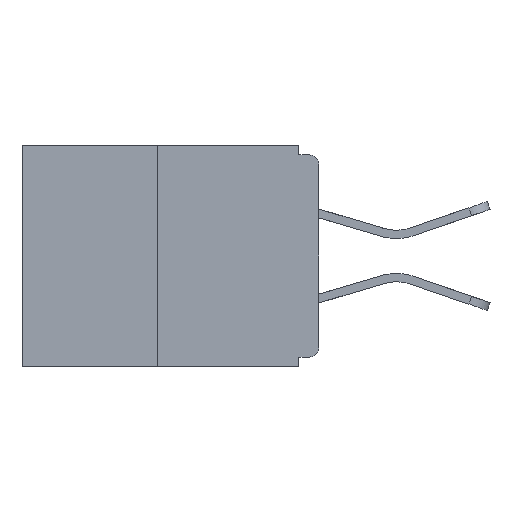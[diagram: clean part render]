
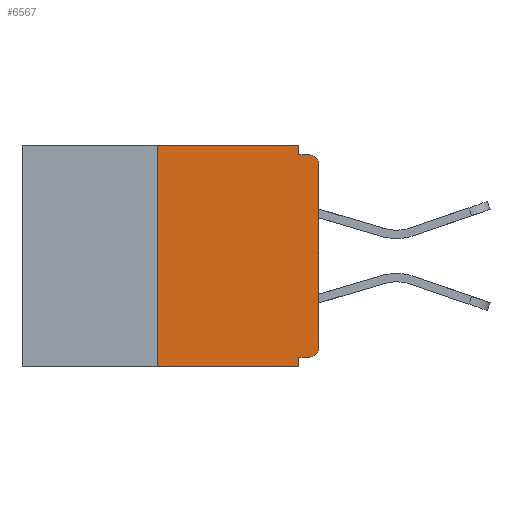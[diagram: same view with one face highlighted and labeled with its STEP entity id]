
A CAD part, left-side view. The second image highlights one B-rep face of the part: STEP entity #6567.
In plain terms, the highlighted planar face has unit normal (-1, 0, 0).
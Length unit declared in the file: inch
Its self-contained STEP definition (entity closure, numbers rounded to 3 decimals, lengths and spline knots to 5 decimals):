
#569 = LINE ( 'NONE', #5429, #4972 ) ;
#860 = LINE ( 'NONE', #4006, #21676 ) ;
#895 = AXIS2_PLACEMENT_3D ( 'NONE', #10374, #14402, #15822 ) ;
#920 = CARTESIAN_POINT ( 'NONE',  ( 0., 0.015, -0.328 ) ) ;
#1297 = ORIENTED_EDGE ( 'NONE', *, *, #5901, .F. ) ;
#1322 = DIRECTION ( 'NONE',  ( 0., 1., 0. ) ) ;
#1736 = DIRECTION ( 'NONE',  ( 0., -1., 0. ) ) ;
#2370 = CARTESIAN_POINT ( 'NONE',  ( 0., 0.031, -0.343 ) ) ;
#2407 = DIRECTION ( 'NONE',  ( 0., 0., 1. ) ) ;
#3159 = ORIENTED_EDGE ( 'NONE', *, *, #17744, .T. ) ;
#3407 = VERTEX_POINT ( 'NONE', #920 ) ;
#3622 = CARTESIAN_POINT ( 'NONE',  ( 0., 0.46, 0. ) ) ;
#4006 = CARTESIAN_POINT ( 'NONE',  ( 0., 0., -0.015 ) ) ;
#4726 = LINE ( 'NONE', #2370, #10388 ) ;
#4780 = CARTESIAN_POINT ( 'NONE',  ( 0., 0.031, -0.328 ) ) ;
#4972 = VECTOR ( 'NONE', #25666, 39.37008 ) ;
#5209 = VERTEX_POINT ( 'NONE', #5967 ) ;
#5330 = ORIENTED_EDGE ( 'NONE', *, *, #9795, .F. ) ;
#5429 = CARTESIAN_POINT ( 'NONE',  ( 0., 0., 0. ) ) ;
#5585 = LINE ( 'NONE', #11495, #7769 ) ;
#5897 = DIRECTION ( 'NONE',  ( 0., -1., 0. ) ) ;
#5901 = EDGE_CURVE ( 'NONE', #5209, #8011, #860, .T. ) ;
#5967 = CARTESIAN_POINT ( 'NONE',  ( 0., 0.031, -0.015 ) ) ;
#6097 = CARTESIAN_POINT ( 'NONE',  ( 0., 0.015, -0.015 ) ) ;
#6567 = ADVANCED_FACE ( 'NONE', ( #22589 ), #18854, .F. ) ;
#6778 = ORIENTED_EDGE ( 'NONE', *, *, #25465, .F. ) ;
#7506 = ORIENTED_EDGE ( 'NONE', *, *, #18424, .F. ) ;
#7606 = AXIS2_PLACEMENT_3D ( 'NONE', #22910, #8778, #23090 ) ;
#7614 = EDGE_CURVE ( 'NONE', #8412, #9125, #20313, .T. ) ;
#7769 = VECTOR ( 'NONE', #21606, 39.37008 ) ;
#8011 = VERTEX_POINT ( 'NONE', #6097 ) ;
#8253 = ORIENTED_EDGE ( 'NONE', *, *, #10452, .F. ) ;
#8412 = VERTEX_POINT ( 'NONE', #9722 ) ;
#8778 = DIRECTION ( 'NONE',  ( 1., 0., 0. ) ) ;
#8795 = CARTESIAN_POINT ( 'NONE',  ( 0., 0.25, 0. ) ) ;
#8951 = CARTESIAN_POINT ( 'NONE',  ( 0., 0.031, 0. ) ) ;
#9125 = VERTEX_POINT ( 'NONE', #23858 ) ;
#9319 = VECTOR ( 'NONE', #1322, 39.37008 ) ;
#9512 = VERTEX_POINT ( 'NONE', #4780 ) ;
#9722 = CARTESIAN_POINT ( 'NONE',  ( 0., 0.25, -0.343 ) ) ;
#9795 = EDGE_CURVE ( 'NONE', #9125, #11968, #23371, .T. ) ;
#10374 = CARTESIAN_POINT ( 'NONE',  ( 0., 0.015, -0.313 ) ) ;
#10388 = VECTOR ( 'NONE', #18570, 39.37008 ) ;
#10452 = EDGE_CURVE ( 'NONE', #9512, #11404, #4726, .T. ) ;
#10732 = CARTESIAN_POINT ( 'NONE',  ( 0., 0., -0.328 ) ) ;
#11404 = VERTEX_POINT ( 'NONE', #15299 ) ;
#11495 = CARTESIAN_POINT ( 'NONE',  ( 0., 0.031, 0. ) ) ;
#11968 = VERTEX_POINT ( 'NONE', #8951 ) ;
#12289 = ORIENTED_EDGE ( 'NONE', *, *, #17236, .T. ) ;
#13171 = CIRCLE ( 'NONE', #16526, 0.015 ) ;
#13923 = CARTESIAN_POINT ( 'NONE',  ( 0., 0., -0.03 ) ) ;
#14402 = DIRECTION ( 'NONE',  ( -1., 0., 0. ) ) ;
#14895 = EDGE_CURVE ( 'NONE', #14925, #8011, #13171, .T. ) ;
#14925 = VERTEX_POINT ( 'NONE', #13923 ) ;
#15299 = CARTESIAN_POINT ( 'NONE',  ( 0., 0.031, -0.343 ) ) ;
#15401 = DIRECTION ( 'NONE',  ( 0., -1., 0. ) ) ;
#15443 = VECTOR ( 'NONE', #5897, 39.37008 ) ;
#15592 = ORIENTED_EDGE ( 'NONE', *, *, #7614, .F. ) ;
#15805 = DIRECTION ( 'NONE',  ( -1., 0., 0. ) ) ;
#15822 = DIRECTION ( 'NONE',  ( 0., 0., -1. ) ) ;
#16526 = AXIS2_PLACEMENT_3D ( 'NONE', #18045, #15805, #19916 ) ;
#17236 = EDGE_CURVE ( 'NONE', #3407, #22325, #20793, .T. ) ;
#17744 = EDGE_CURVE ( 'NONE', #22325, #14925, #569, .T. ) ;
#18045 = CARTESIAN_POINT ( 'NONE',  ( 0., 0.015, -0.03 ) ) ;
#18424 = EDGE_CURVE ( 'NONE', #3407, #9512, #19757, .T. ) ;
#18570 = DIRECTION ( 'NONE',  ( 0., 0., -1. ) ) ;
#18854 = PLANE ( 'NONE',  #7606 ) ;
#19009 = VECTOR ( 'NONE', #2407, 39.37008 ) ;
#19250 = CARTESIAN_POINT ( 'NONE',  ( 0., 0., -0.313 ) ) ;
#19757 = LINE ( 'NONE', #10732, #9319 ) ;
#19842 = ORIENTED_EDGE ( 'NONE', *, *, #22861, .T. ) ;
#19894 = EDGE_LOOP ( 'NONE', ( #5330, #15592, #19842, #8253, #7506, #12289, #3159, #21653, #1297, #6778 ) ) ;
#19916 = DIRECTION ( 'NONE',  ( 0., 0., -1. ) ) ;
#20313 = LINE ( 'NONE', #8795, #19009 ) ;
#20793 = CIRCLE ( 'NONE', #895, 0.015 ) ;
#21606 = DIRECTION ( 'NONE',  ( 0., 0., -1. ) ) ;
#21653 = ORIENTED_EDGE ( 'NONE', *, *, #14895, .T. ) ;
#21676 = VECTOR ( 'NONE', #1736, 39.37008 ) ;
#22325 = VERTEX_POINT ( 'NONE', #19250 ) ;
#22589 = FACE_OUTER_BOUND ( 'NONE', #19894, .T. ) ;
#22861 = EDGE_CURVE ( 'NONE', #8412, #11404, #22991, .T. ) ;
#22910 = CARTESIAN_POINT ( 'NONE',  ( 0., 0.46, 0. ) ) ;
#22991 = LINE ( 'NONE', #25346, #25225 ) ;
#23090 = DIRECTION ( 'NONE',  ( 0., 0., -1. ) ) ;
#23371 = LINE ( 'NONE', #3622, #15443 ) ;
#23858 = CARTESIAN_POINT ( 'NONE',  ( 0., 0.25, 0. ) ) ;
#25225 = VECTOR ( 'NONE', #15401, 39.37008 ) ;
#25346 = CARTESIAN_POINT ( 'NONE',  ( 0., 0.46, -0.343 ) ) ;
#25465 = EDGE_CURVE ( 'NONE', #11968, #5209, #5585, .T. ) ;
#25666 = DIRECTION ( 'NONE',  ( 0., 0., 1. ) ) ;
